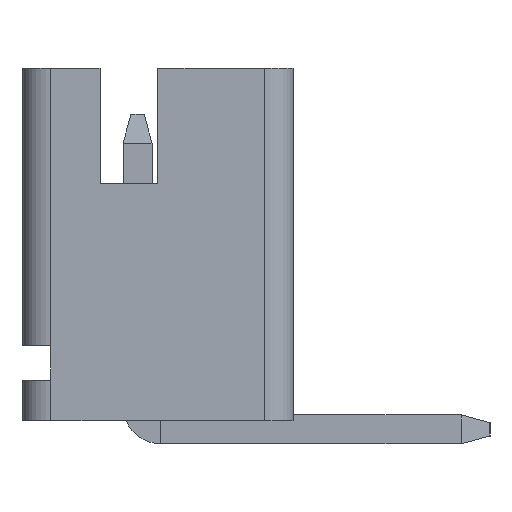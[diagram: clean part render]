
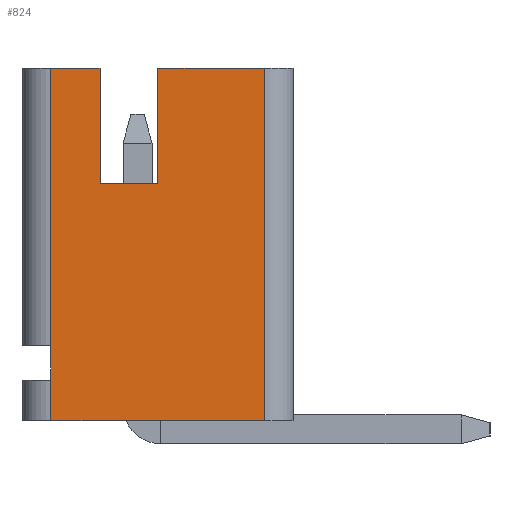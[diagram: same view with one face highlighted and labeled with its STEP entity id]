
A CAD part, left-side view. The second image highlights one B-rep face of the part: STEP entity #824.
In plain terms, the highlighted planar face has unit normal (-1, 0, 0).
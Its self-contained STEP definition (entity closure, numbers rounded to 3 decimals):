
#14 = VERTEX_POINT ( 'NONE', #388 ) ;
#152 = EDGE_CURVE ( 'NONE', #1459, #2100, #4128, .T. ) ;
#284 = VECTOR ( 'NONE', #2047, 1000. ) ;
#307 = VECTOR ( 'NONE', #2154, 1000. ) ;
#388 = CARTESIAN_POINT ( 'NONE',  ( -2., -0.35, 6.1 ) ) ;
#582 = CARTESIAN_POINT ( 'NONE',  ( -2., 0., 0. ) ) ;
#691 = EDGE_CURVE ( 'NONE', #4349, #3868, #5328, .T. ) ;
#693 = CARTESIAN_POINT ( 'NONE',  ( -2., -2.2, 0. ) ) ;
#780 = LINE ( 'NONE', #5657, #5258 ) ;
#824 = ADVANCED_FACE ( 'NONE', ( #4834 ), #854, .T. ) ;
#854 = PLANE ( 'NONE',  #4139 ) ;
#970 = CARTESIAN_POINT ( 'NONE',  ( -2., 1.5, 6.1 ) ) ;
#1020 = DIRECTION ( 'NONE',  ( 0., 0., -1. ) ) ;
#1092 = LINE ( 'NONE', #4280, #284 ) ;
#1131 = EDGE_CURVE ( 'NONE', #5189, #14, #1802, .T. ) ;
#1313 = ORIENTED_EDGE ( 'NONE', *, *, #691, .T. ) ;
#1319 = VECTOR ( 'NONE', #1346, 1000. ) ;
#1346 = DIRECTION ( 'NONE',  ( 0., 0., 1. ) ) ;
#1459 = VERTEX_POINT ( 'NONE', #3451 ) ;
#1468 = VERTEX_POINT ( 'NONE', #693 ) ;
#1499 = EDGE_CURVE ( 'NONE', #2998, #4349, #780, .T. ) ;
#1666 = LINE ( 'NONE', #3439, #1319 ) ;
#1693 = EDGE_LOOP ( 'NONE', ( #2306, #2612, #4671, #5223, #5471, #1313, #4650, #2654, #2599, #2022 ) ) ;
#1769 = VERTEX_POINT ( 'NONE', #970 ) ;
#1802 = LINE ( 'NONE', #3137, #1822 ) ;
#1822 = VECTOR ( 'NONE', #4386, 1000. ) ;
#2022 = ORIENTED_EDGE ( 'NONE', *, *, #152, .T. ) ;
#2047 = DIRECTION ( 'NONE',  ( 0., -1., 0. ) ) ;
#2067 = LINE ( 'NONE', #2585, #2773 ) ;
#2100 = VERTEX_POINT ( 'NONE', #2596 ) ;
#2137 = CARTESIAN_POINT ( 'NONE',  ( -2., -2.2, 6.1 ) ) ;
#2154 = DIRECTION ( 'NONE',  ( 0., 0., -1. ) ) ;
#2212 = EDGE_CURVE ( 'NONE', #1468, #5189, #1666, .T. ) ;
#2306 = ORIENTED_EDGE ( 'NONE', *, *, #4585, .T. ) ;
#2327 = DIRECTION ( 'NONE',  ( 0., 0., -1. ) ) ;
#2530 = CARTESIAN_POINT ( 'NONE',  ( -2., 2., 6.1 ) ) ;
#2585 = CARTESIAN_POINT ( 'NONE',  ( -2., -0.35, 6.1 ) ) ;
#2596 = CARTESIAN_POINT ( 'NONE',  ( -2., 1.5, 0. ) ) ;
#2599 = ORIENTED_EDGE ( 'NONE', *, *, #5488, .T. ) ;
#2600 = CARTESIAN_POINT ( 'NONE',  ( -2., 0.65, 6.1 ) ) ;
#2608 = EDGE_CURVE ( 'NONE', #14, #2998, #2067, .T. ) ;
#2612 = ORIENTED_EDGE ( 'NONE', *, *, #2212, .T. ) ;
#2654 = ORIENTED_EDGE ( 'NONE', *, *, #4807, .T. ) ;
#2773 = VECTOR ( 'NONE', #3505, 1000. ) ;
#2998 = VERTEX_POINT ( 'NONE', #4154 ) ;
#3137 = CARTESIAN_POINT ( 'NONE',  ( -2., -0.35, 6.1 ) ) ;
#3294 = LINE ( 'NONE', #2530, #3925 ) ;
#3432 = VERTEX_POINT ( 'NONE', #3486 ) ;
#3439 = CARTESIAN_POINT ( 'NONE',  ( -2., -2.2, 0. ) ) ;
#3451 = CARTESIAN_POINT ( 'NONE',  ( -2., 1.5, 0.7 ) ) ;
#3486 = CARTESIAN_POINT ( 'NONE',  ( -2., 1.5, 1.3 ) ) ;
#3505 = DIRECTION ( 'NONE',  ( 0., 0., -1. ) ) ;
#3711 = VECTOR ( 'NONE', #2327, 1000. ) ;
#3800 = DIRECTION ( 'NONE',  ( 0., 1., 0. ) ) ;
#3868 = VERTEX_POINT ( 'NONE', #5687 ) ;
#3925 = VECTOR ( 'NONE', #5179, 1000. ) ;
#4125 = DIRECTION ( 'NONE',  ( 0., -1., 0. ) ) ;
#4128 = LINE ( 'NONE', #4589, #4656 ) ;
#4139 = AXIS2_PLACEMENT_3D ( 'NONE', #582, #5523, #4125 ) ;
#4154 = CARTESIAN_POINT ( 'NONE',  ( -2., -0.35, 4.1 ) ) ;
#4280 = CARTESIAN_POINT ( 'NONE',  ( -2., 2., 0. ) ) ;
#4349 = VERTEX_POINT ( 'NONE', #4896 ) ;
#4358 = LINE ( 'NONE', #4797, #307 ) ;
#4386 = DIRECTION ( 'NONE',  ( 0., 1., 0. ) ) ;
#4414 = VECTOR ( 'NONE', #5272, 1000. ) ;
#4526 = CARTESIAN_POINT ( 'NONE',  ( -2., 1.5, 0. ) ) ;
#4585 = EDGE_CURVE ( 'NONE', #2100, #1468, #1092, .T. ) ;
#4589 = CARTESIAN_POINT ( 'NONE',  ( -2., 1.5, 0. ) ) ;
#4650 = ORIENTED_EDGE ( 'NONE', *, *, #5457, .T. ) ;
#4656 = VECTOR ( 'NONE', #1020, 1000. ) ;
#4671 = ORIENTED_EDGE ( 'NONE', *, *, #1131, .T. ) ;
#4797 = CARTESIAN_POINT ( 'NONE',  ( -2., 1.5, 1.3 ) ) ;
#4807 = EDGE_CURVE ( 'NONE', #1769, #3432, #4964, .T. ) ;
#4834 = FACE_OUTER_BOUND ( 'NONE', #1693, .T. ) ;
#4896 = CARTESIAN_POINT ( 'NONE',  ( -2., 0.65, 4.1 ) ) ;
#4964 = LINE ( 'NONE', #4526, #3711 ) ;
#5179 = DIRECTION ( 'NONE',  ( 0., 1., 0. ) ) ;
#5189 = VERTEX_POINT ( 'NONE', #2137 ) ;
#5223 = ORIENTED_EDGE ( 'NONE', *, *, #2608, .T. ) ;
#5258 = VECTOR ( 'NONE', #3800, 1000. ) ;
#5272 = DIRECTION ( 'NONE',  ( 0., 0., 1. ) ) ;
#5328 = LINE ( 'NONE', #2600, #4414 ) ;
#5457 = EDGE_CURVE ( 'NONE', #3868, #1769, #3294, .T. ) ;
#5471 = ORIENTED_EDGE ( 'NONE', *, *, #1499, .T. ) ;
#5488 = EDGE_CURVE ( 'NONE', #3432, #1459, #4358, .T. ) ;
#5523 = DIRECTION ( 'NONE',  ( -1., 0., 0. ) ) ;
#5657 = CARTESIAN_POINT ( 'NONE',  ( -2., 0.65, 4.1 ) ) ;
#5687 = CARTESIAN_POINT ( 'NONE',  ( -2., 0.65, 6.1 ) ) ;
